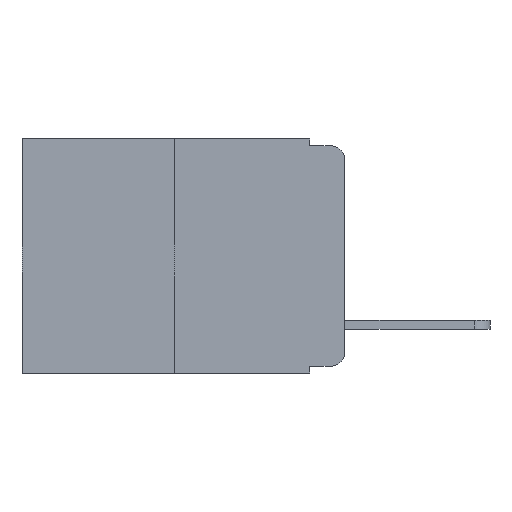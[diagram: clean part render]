
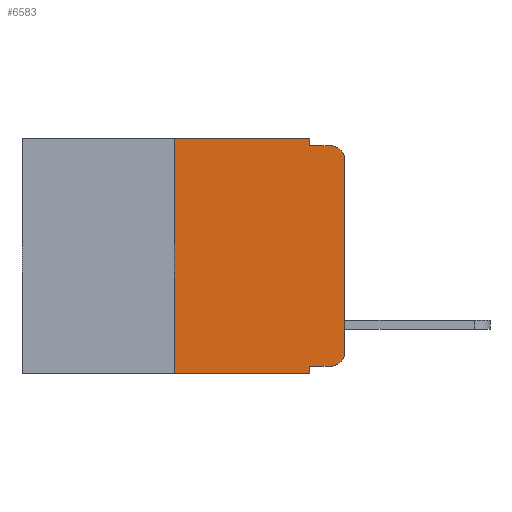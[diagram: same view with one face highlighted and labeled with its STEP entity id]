
A CAD part, left-side view. The second image highlights one B-rep face of the part: STEP entity #6583.
In plain terms, the highlighted planar face has unit normal (-1, 0, 0).
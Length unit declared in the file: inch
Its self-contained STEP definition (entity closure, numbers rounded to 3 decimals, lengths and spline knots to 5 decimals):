
#6 = AXIS2_PLACEMENT_3D ( 'NONE', #12550, #1963, #14284 ) ;
#330 = CIRCLE ( 'NONE', #6, 0.02 ) ;
#582 = ORIENTED_EDGE ( 'NONE', *, *, #15911, .T. ) ;
#688 = CARTESIAN_POINT ( 'NONE',  ( 0., 0.473, -0.343 ) ) ;
#1518 = VERTEX_POINT ( 'NONE', #21675 ) ;
#1592 = VERTEX_POINT ( 'NONE', #12906 ) ;
#1963 = DIRECTION ( 'NONE',  ( -1., 0., 0. ) ) ;
#2556 = EDGE_CURVE ( 'NONE', #3797, #17457, #11364, .T. ) ;
#2814 = EDGE_CURVE ( 'NONE', #21778, #13669, #16216, .T. ) ;
#3187 = ORIENTED_EDGE ( 'NONE', *, *, #16596, .T. ) ;
#3229 = CIRCLE ( 'NONE', #8331, 0.02 ) ;
#3797 = VERTEX_POINT ( 'NONE', #7302 ) ;
#4402 = ORIENTED_EDGE ( 'NONE', *, *, #7126, .T. ) ;
#4607 = CARTESIAN_POINT ( 'NONE',  ( 0., 0.051, -0.333 ) ) ;
#4681 = VERTEX_POINT ( 'NONE', #6109 ) ;
#5016 = LINE ( 'NONE', #4607, #18239 ) ;
#5229 = CARTESIAN_POINT ( 'NONE',  ( 0., 0.473, 0. ) ) ;
#6109 = CARTESIAN_POINT ( 'NONE',  ( 0., 0.051, -0.333 ) ) ;
#6161 = CARTESIAN_POINT ( 'NONE',  ( 0., 0.051, -0.01 ) ) ;
#6388 = EDGE_CURVE ( 'NONE', #1592, #21523, #18993, .T. ) ;
#6583 = ADVANCED_FACE ( 'NONE', ( #9635 ), #15670, .F. ) ;
#6597 = DIRECTION ( 'NONE',  ( 0., 0., -1. ) ) ;
#6715 = VERTEX_POINT ( 'NONE', #20989 ) ;
#6827 = DIRECTION ( 'NONE',  ( 0., 0., 1. ) ) ;
#7126 = EDGE_CURVE ( 'NONE', #1518, #6715, #17122, .T. ) ;
#7302 = CARTESIAN_POINT ( 'NONE',  ( 0., 0.25, -0.343 ) ) ;
#7694 = DIRECTION ( 'NONE',  ( -1., 0., 0. ) ) ;
#8068 = EDGE_CURVE ( 'NONE', #3797, #21778, #20490, .T. ) ;
#8245 = VERTEX_POINT ( 'NONE', #9542 ) ;
#8331 = AXIS2_PLACEMENT_3D ( 'NONE', #17998, #7694, #19677 ) ;
#8468 = ORIENTED_EDGE ( 'NONE', *, *, #2814, .F. ) ;
#8513 = CARTESIAN_POINT ( 'NONE',  ( 0., 0., 0. ) ) ;
#8764 = DIRECTION ( 'NONE',  ( 0., 0., -1. ) ) ;
#9194 = CARTESIAN_POINT ( 'NONE',  ( 0., 0.25, 0. ) ) ;
#9542 = CARTESIAN_POINT ( 'NONE',  ( 0., 0.02, -0.333 ) ) ;
#9635 = FACE_OUTER_BOUND ( 'NONE', #13518, .T. ) ;
#9895 = DIRECTION ( 'NONE',  ( 0., -1., 0. ) ) ;
#10020 = CARTESIAN_POINT ( 'NONE',  ( 0., 0.051, 0. ) ) ;
#10135 = VECTOR ( 'NONE', #6597, 39.37008 ) ;
#10307 = AXIS2_PLACEMENT_3D ( 'NONE', #5229, #19002, #8764 ) ;
#10548 = ORIENTED_EDGE ( 'NONE', *, *, #2556, .T. ) ;
#10778 = CARTESIAN_POINT ( 'NONE',  ( 0., 0.25, 0. ) ) ;
#10822 = VECTOR ( 'NONE', #19615, 39.37008 ) ;
#11312 = CARTESIAN_POINT ( 'NONE',  ( 0., 0.051, 0. ) ) ;
#11364 = LINE ( 'NONE', #688, #10822 ) ;
#12059 = VECTOR ( 'NONE', #6827, 39.37008 ) ;
#12260 = CARTESIAN_POINT ( 'NONE',  ( 0., 0.02, -0.01 ) ) ;
#12550 = CARTESIAN_POINT ( 'NONE',  ( 0., 0.02, -0.313 ) ) ;
#12681 = CARTESIAN_POINT ( 'NONE',  ( 0., 0.051, -0.343 ) ) ;
#12906 = CARTESIAN_POINT ( 'NONE',  ( 0., 0.051, -0.01 ) ) ;
#13506 = CARTESIAN_POINT ( 'NONE',  ( 0., 0.473, 0. ) ) ;
#13518 = EDGE_LOOP ( 'NONE', ( #4402, #16372, #17927, #14524, #8468, #17825, #10548, #13796, #3187, #582 ) ) ;
#13669 = VERTEX_POINT ( 'NONE', #11312 ) ;
#13796 = ORIENTED_EDGE ( 'NONE', *, *, #19947, .F. ) ;
#14004 = VECTOR ( 'NONE', #21590, 39.37008 ) ;
#14265 = DIRECTION ( 'NONE',  ( 0., 0., 1. ) ) ;
#14284 = DIRECTION ( 'NONE',  ( 0., 0., -1. ) ) ;
#14524 = ORIENTED_EDGE ( 'NONE', *, *, #18399, .F. ) ;
#14782 = LINE ( 'NONE', #10020, #10135 ) ;
#15670 = PLANE ( 'NONE',  #10307 ) ;
#15911 = EDGE_CURVE ( 'NONE', #8245, #1518, #330, .T. ) ;
#16066 = VECTOR ( 'NONE', #14265, 39.37008 ) ;
#16216 = LINE ( 'NONE', #13506, #19581 ) ;
#16372 = ORIENTED_EDGE ( 'NONE', *, *, #19041, .T. ) ;
#16596 = EDGE_CURVE ( 'NONE', #4681, #8245, #5016, .T. ) ;
#16603 = VECTOR ( 'NONE', #22219, 39.37008 ) ;
#17122 = LINE ( 'NONE', #8513, #12059 ) ;
#17457 = VERTEX_POINT ( 'NONE', #12681 ) ;
#17825 = ORIENTED_EDGE ( 'NONE', *, *, #8068, .F. ) ;
#17927 = ORIENTED_EDGE ( 'NONE', *, *, #6388, .F. ) ;
#17998 = CARTESIAN_POINT ( 'NONE',  ( 0., 0.02, -0.03 ) ) ;
#18239 = VECTOR ( 'NONE', #9895, 39.37008 ) ;
#18399 = EDGE_CURVE ( 'NONE', #13669, #1592, #21577, .T. ) ;
#18993 = LINE ( 'NONE', #6161, #14004 ) ;
#19002 = DIRECTION ( 'NONE',  ( 1., 0., 0. ) ) ;
#19041 = EDGE_CURVE ( 'NONE', #6715, #21523, #3229, .T. ) ;
#19549 = DIRECTION ( 'NONE',  ( 0., -1., 0. ) ) ;
#19581 = VECTOR ( 'NONE', #19549, 39.37008 ) ;
#19615 = DIRECTION ( 'NONE',  ( 0., -1., 0. ) ) ;
#19677 = DIRECTION ( 'NONE',  ( 0., 0., -1. ) ) ;
#19947 = EDGE_CURVE ( 'NONE', #4681, #17457, #14782, .T. ) ;
#20490 = LINE ( 'NONE', #10778, #16066 ) ;
#20543 = CARTESIAN_POINT ( 'NONE',  ( 0., 0.051, 0. ) ) ;
#20989 = CARTESIAN_POINT ( 'NONE',  ( 0., 0., -0.03 ) ) ;
#21523 = VERTEX_POINT ( 'NONE', #12260 ) ;
#21577 = LINE ( 'NONE', #20543, #16603 ) ;
#21590 = DIRECTION ( 'NONE',  ( 0., -1., 0. ) ) ;
#21675 = CARTESIAN_POINT ( 'NONE',  ( 0., 0., -0.313 ) ) ;
#21778 = VERTEX_POINT ( 'NONE', #9194 ) ;
#22219 = DIRECTION ( 'NONE',  ( 0., 0., -1. ) ) ;
